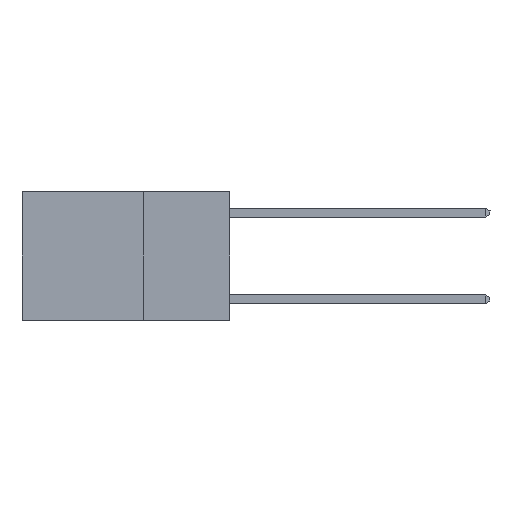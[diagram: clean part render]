
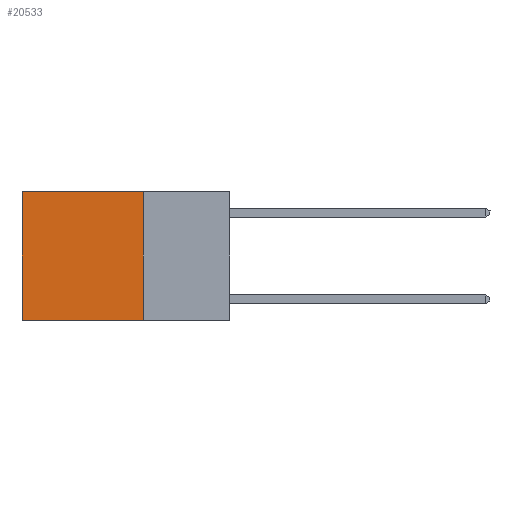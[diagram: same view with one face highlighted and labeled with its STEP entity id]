
A CAD part, left-side view. The second image highlights one B-rep face of the part: STEP entity #20533.
In plain terms, the highlighted planar face has unit normal (-1, 0, 0).
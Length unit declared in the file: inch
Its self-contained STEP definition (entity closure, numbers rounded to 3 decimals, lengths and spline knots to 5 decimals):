
#165 = ORIENTED_EDGE ( 'NONE', *, *, #9142, .T. ) ;
#1440 = DIRECTION ( 'NONE',  ( 0., 1., 0. ) ) ;
#1771 = VECTOR ( 'NONE', #30636, 39.37008 ) ;
#7813 = VECTOR ( 'NONE', #1440, 39.37008 ) ;
#8816 = CARTESIAN_POINT ( 'NONE',  ( 0.2625, 0.25, 0. ) ) ;
#8914 = EDGE_CURVE ( 'NONE', #17776, #22003, #11828, .T. ) ;
#9006 = EDGE_CURVE ( 'NONE', #10033, #18172, #10099, .T. ) ;
#9142 = EDGE_CURVE ( 'NONE', #17776, #10033, #25576, .T. ) ;
#9292 = DIRECTION ( 'NONE',  ( 1., 0., 0. ) ) ;
#9475 = CARTESIAN_POINT ( 'NONE',  ( 0.2625, 0.25, 0. ) ) ;
#9950 = DIRECTION ( 'NONE',  ( 0., 0., -1. ) ) ;
#10033 = VERTEX_POINT ( 'NONE', #17550 ) ;
#10099 = LINE ( 'NONE', #12761, #17852 ) ;
#11828 = LINE ( 'NONE', #9475, #1771 ) ;
#12761 = CARTESIAN_POINT ( 'NONE',  ( 0.2625, 0.6, 0. ) ) ;
#16115 = CARTESIAN_POINT ( 'NONE',  ( 0.2625, 0.25, -0.37 ) ) ;
#16150 = ORIENTED_EDGE ( 'NONE', *, *, #9006, .T. ) ;
#16841 = DIRECTION ( 'NONE',  ( 0., 0., -1. ) ) ;
#16857 = ORIENTED_EDGE ( 'NONE', *, *, #29950, .F. ) ;
#17013 = PLANE ( 'NONE',  #18917 ) ;
#17088 = ORIENTED_EDGE ( 'NONE', *, *, #8914, .F. ) ;
#17550 = CARTESIAN_POINT ( 'NONE',  ( 0.2625, 0.6, 0. ) ) ;
#17776 = VERTEX_POINT ( 'NONE', #29097 ) ;
#17852 = VECTOR ( 'NONE', #9950, 39.37008 ) ;
#18172 = VERTEX_POINT ( 'NONE', #26197 ) ;
#18903 = CARTESIAN_POINT ( 'NONE',  ( 0.2625, 0.25, 0. ) ) ;
#18917 = AXIS2_PLACEMENT_3D ( 'NONE', #18903, #9292, #16841 ) ;
#19526 = FACE_OUTER_BOUND ( 'NONE', #27859, .T. ) ;
#20533 = ADVANCED_FACE ( 'NONE', ( #19526 ), #17013, .F. ) ;
#20843 = VECTOR ( 'NONE', #20976, 39.37008 ) ;
#20976 = DIRECTION ( 'NONE',  ( 0., 1., 0. ) ) ;
#22003 = VERTEX_POINT ( 'NONE', #28579 ) ;
#25576 = LINE ( 'NONE', #8816, #7813 ) ;
#26197 = CARTESIAN_POINT ( 'NONE',  ( 0.2625, 0.6, -0.37 ) ) ;
#27859 = EDGE_LOOP ( 'NONE', ( #16150, #16857, #17088, #165 ) ) ;
#28579 = CARTESIAN_POINT ( 'NONE',  ( 0.2625, 0.25, -0.37 ) ) ;
#29097 = CARTESIAN_POINT ( 'NONE',  ( 0.2625, 0.25, 0. ) ) ;
#29950 = EDGE_CURVE ( 'NONE', #22003, #18172, #30044, .T. ) ;
#30044 = LINE ( 'NONE', #16115, #20843 ) ;
#30636 = DIRECTION ( 'NONE',  ( 0., 0., -1. ) ) ;
